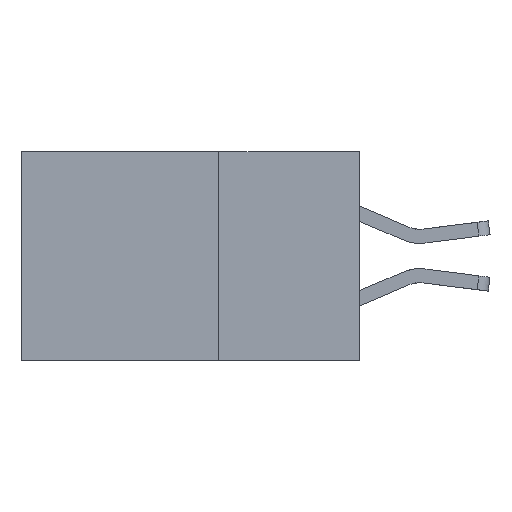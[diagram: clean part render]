
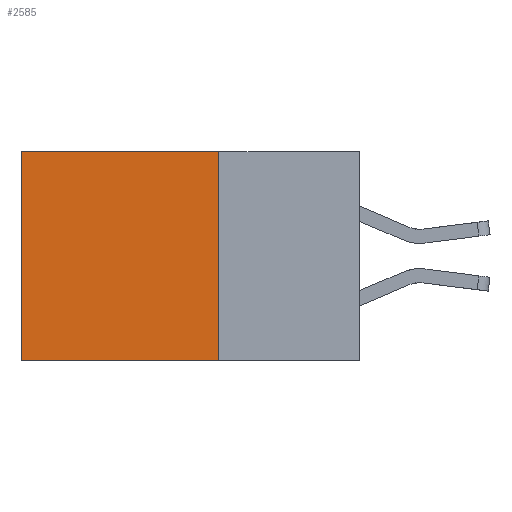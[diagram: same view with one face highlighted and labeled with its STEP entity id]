
A CAD part, left-side view. The second image highlights one B-rep face of the part: STEP entity #2585.
In plain terms, the highlighted planar face has unit normal (-1, 0, 0).
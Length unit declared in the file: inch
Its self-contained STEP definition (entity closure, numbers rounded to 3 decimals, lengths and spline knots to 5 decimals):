
#326 = CARTESIAN_POINT ( 'NONE',  ( 0.2875, 0.25, 0. ) ) ;
#623 = CARTESIAN_POINT ( 'NONE',  ( 0.2875, 0.25, 0. ) ) ;
#721 = DIRECTION ( 'NONE',  ( 0., 1., 0. ) ) ;
#890 = ORIENTED_EDGE ( 'NONE', *, *, #13344, .F. ) ;
#934 = CARTESIAN_POINT ( 'NONE',  ( 0.2875, 0.6, 0. ) ) ;
#1376 = ORIENTED_EDGE ( 'NONE', *, *, #8970, .T. ) ;
#2585 = ADVANCED_FACE ( 'NONE', ( #12003 ), #5808, .F. ) ;
#4345 = CARTESIAN_POINT ( 'NONE',  ( 0.2875, 0.25, 0. ) ) ;
#5554 = VECTOR ( 'NONE', #7945, 39.37008 ) ;
#5733 = CARTESIAN_POINT ( 'NONE',  ( 0.2875, 0.25, -0.37 ) ) ;
#5808 = PLANE ( 'NONE',  #9977 ) ;
#5895 = LINE ( 'NONE', #6832, #5554 ) ;
#6813 = DIRECTION ( 'NONE',  ( 0., 0., -1. ) ) ;
#6832 = CARTESIAN_POINT ( 'NONE',  ( 0.2875, 0.25, -0.37 ) ) ;
#7616 = VECTOR ( 'NONE', #6813, 39.37008 ) ;
#7673 = ORIENTED_EDGE ( 'NONE', *, *, #10098, .T. ) ;
#7854 = EDGE_LOOP ( 'NONE', ( #7673, #12286, #890, #1376 ) ) ;
#7945 = DIRECTION ( 'NONE',  ( 0., 1., 0. ) ) ;
#7947 = VECTOR ( 'NONE', #721, 39.37008 ) ;
#8607 = DIRECTION ( 'NONE',  ( 0., 0., -1. ) ) ;
#8700 = VERTEX_POINT ( 'NONE', #5733 ) ;
#8970 = EDGE_CURVE ( 'NONE', #9389, #11336, #13483, .T. ) ;
#9389 = VERTEX_POINT ( 'NONE', #4345 ) ;
#9977 = AXIS2_PLACEMENT_3D ( 'NONE', #10435, #10384, #10805 ) ;
#10069 = VERTEX_POINT ( 'NONE', #10753 ) ;
#10098 = EDGE_CURVE ( 'NONE', #11336, #10069, #13110, .T. ) ;
#10384 = DIRECTION ( 'NONE',  ( 1., 0., 0. ) ) ;
#10386 = VECTOR ( 'NONE', #8607, 39.37008 ) ;
#10435 = CARTESIAN_POINT ( 'NONE',  ( 0.2875, 0.25, 0. ) ) ;
#10753 = CARTESIAN_POINT ( 'NONE',  ( 0.2875, 0.6, -0.37 ) ) ;
#10805 = DIRECTION ( 'NONE',  ( 0., 0., -1. ) ) ;
#10808 = LINE ( 'NONE', #326, #7616 ) ;
#11336 = VERTEX_POINT ( 'NONE', #934 ) ;
#12003 = FACE_OUTER_BOUND ( 'NONE', #7854, .T. ) ;
#12286 = ORIENTED_EDGE ( 'NONE', *, *, #12319, .F. ) ;
#12319 = EDGE_CURVE ( 'NONE', #8700, #10069, #5895, .T. ) ;
#12796 = CARTESIAN_POINT ( 'NONE',  ( 0.2875, 0.6, 0. ) ) ;
#13110 = LINE ( 'NONE', #12796, #10386 ) ;
#13344 = EDGE_CURVE ( 'NONE', #9389, #8700, #10808, .T. ) ;
#13483 = LINE ( 'NONE', #623, #7947 ) ;
